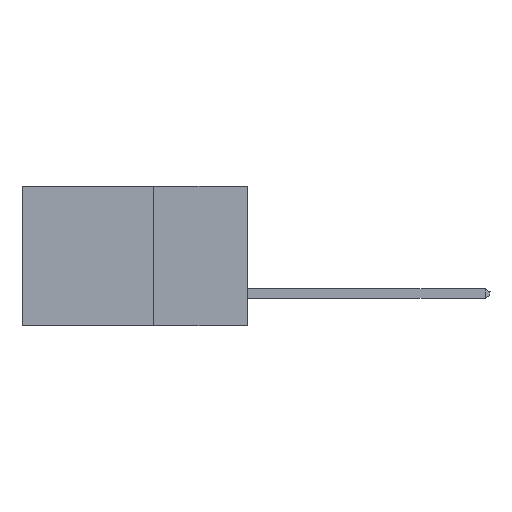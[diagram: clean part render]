
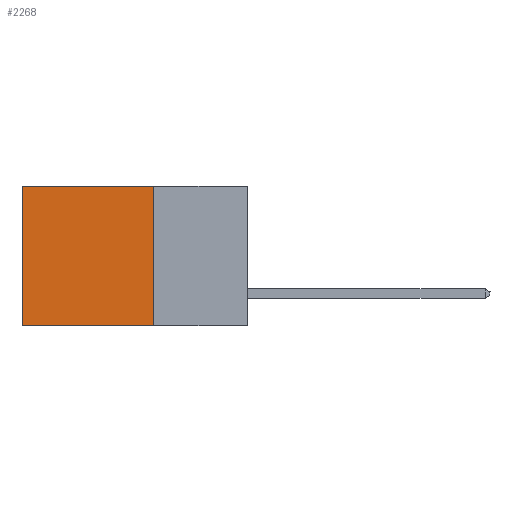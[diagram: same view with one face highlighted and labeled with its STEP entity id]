
A CAD part, left-side view. The second image highlights one B-rep face of the part: STEP entity #2268.
In plain terms, the highlighted planar face has unit normal (-1, 0, 0).
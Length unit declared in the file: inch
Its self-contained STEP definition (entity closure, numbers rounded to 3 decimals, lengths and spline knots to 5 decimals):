
#83 = VECTOR ( 'NONE', #5048, 39.37008 ) ;
#1432 = CARTESIAN_POINT ( 'NONE',  ( 0.2615, 0.25, -0.37 ) ) ;
#2028 = LINE ( 'NONE', #5917, #83 ) ;
#2268 = ADVANCED_FACE ( 'NONE', ( #9518 ), #5627, .F. ) ;
#2707 = CARTESIAN_POINT ( 'NONE',  ( 0.2615, 0.25, 0. ) ) ;
#2861 = DIRECTION ( 'NONE',  ( 0., 0., -1. ) ) ;
#2928 = ORIENTED_EDGE ( 'NONE', *, *, #9469, .T. ) ;
#3225 = CARTESIAN_POINT ( 'NONE',  ( 0.2615, 0.25, -0.37 ) ) ;
#3257 = CARTESIAN_POINT ( 'NONE',  ( 0.2615, 0.6, -0.37 ) ) ;
#3633 = VECTOR ( 'NONE', #9885, 39.37008 ) ;
#4275 = LINE ( 'NONE', #1432, #3633 ) ;
#4999 = EDGE_LOOP ( 'NONE', ( #10956, #10349, #9573, #2928 ) ) ;
#5048 = DIRECTION ( 'NONE',  ( 0., 0., -1. ) ) ;
#5627 = PLANE ( 'NONE',  #6097 ) ;
#5665 = CARTESIAN_POINT ( 'NONE',  ( 0.2615, 0.25, 0. ) ) ;
#5917 = CARTESIAN_POINT ( 'NONE',  ( 0.2615, 0.6, -0.37 ) ) ;
#5929 = EDGE_CURVE ( 'NONE', #9569, #7123, #7681, .T. ) ;
#6067 = DIRECTION ( 'NONE',  ( 0., 0., -1. ) ) ;
#6097 = AXIS2_PLACEMENT_3D ( 'NONE', #7552, #9580, #2861 ) ;
#6776 = CARTESIAN_POINT ( 'NONE',  ( 0.2615, 0.6, 0. ) ) ;
#7123 = VERTEX_POINT ( 'NONE', #8914 ) ;
#7181 = VECTOR ( 'NONE', #8085, 39.37008 ) ;
#7552 = CARTESIAN_POINT ( 'NONE',  ( 0.2615, 0.25, -0.37 ) ) ;
#7681 = LINE ( 'NONE', #3225, #11471 ) ;
#8062 = EDGE_CURVE ( 'NONE', #9084, #9704, #2028, .T. ) ;
#8085 = DIRECTION ( 'NONE',  ( 0., 1., 0. ) ) ;
#8438 = EDGE_CURVE ( 'NONE', #7123, #9704, #4275, .T. ) ;
#8914 = CARTESIAN_POINT ( 'NONE',  ( 0.2615, 0.25, -0.37 ) ) ;
#9084 = VERTEX_POINT ( 'NONE', #6776 ) ;
#9469 = EDGE_CURVE ( 'NONE', #9569, #9084, #11158, .T. ) ;
#9518 = FACE_OUTER_BOUND ( 'NONE', #4999, .T. ) ;
#9569 = VERTEX_POINT ( 'NONE', #5665 ) ;
#9573 = ORIENTED_EDGE ( 'NONE', *, *, #5929, .F. ) ;
#9580 = DIRECTION ( 'NONE',  ( 1., 0., 0. ) ) ;
#9704 = VERTEX_POINT ( 'NONE', #3257 ) ;
#9885 = DIRECTION ( 'NONE',  ( 0., 1., 0. ) ) ;
#10349 = ORIENTED_EDGE ( 'NONE', *, *, #8438, .F. ) ;
#10956 = ORIENTED_EDGE ( 'NONE', *, *, #8062, .T. ) ;
#11158 = LINE ( 'NONE', #2707, #7181 ) ;
#11471 = VECTOR ( 'NONE', #6067, 39.37008 ) ;
